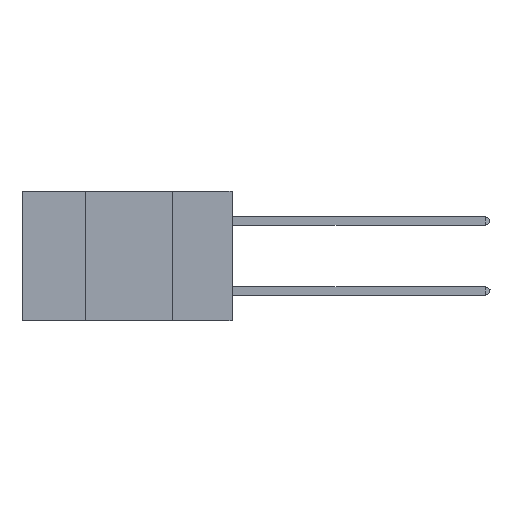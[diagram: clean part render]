
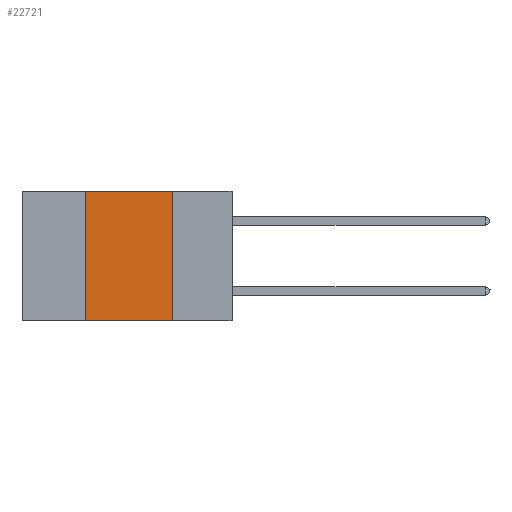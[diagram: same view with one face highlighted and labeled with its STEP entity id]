
A CAD part, left-side view. The second image highlights one B-rep face of the part: STEP entity #22721.
In plain terms, the highlighted planar face has unit normal (-1, 0, 0).
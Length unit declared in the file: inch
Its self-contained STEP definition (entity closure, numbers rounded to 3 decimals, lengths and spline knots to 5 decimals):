
#283 = PLANE ( 'NONE',  #12346 ) ;
#873 = DIRECTION ( 'NONE',  ( 0., 0., -1. ) ) ;
#2026 = VECTOR ( 'NONE', #14570, 39.37008 ) ;
#3414 = VERTEX_POINT ( 'NONE', #14334 ) ;
#3845 = ORIENTED_EDGE ( 'NONE', *, *, #28315, .F. ) ;
#4107 = ORIENTED_EDGE ( 'NONE', *, *, #23686, .F. ) ;
#4733 = CARTESIAN_POINT ( 'NONE',  ( 0., 0.6, 0. ) ) ;
#4884 = EDGE_CURVE ( 'NONE', #3414, #23263, #25517, .T. ) ;
#5746 = DIRECTION ( 'NONE',  ( 0., 0., 1. ) ) ;
#6227 = CARTESIAN_POINT ( 'NONE',  ( 0., 0.17, 0. ) ) ;
#6267 = VECTOR ( 'NONE', #20473, 39.37008 ) ;
#7265 = CARTESIAN_POINT ( 'NONE',  ( 0., 0.17, -0.37 ) ) ;
#7806 = LINE ( 'NONE', #25553, #24580 ) ;
#7925 = ORIENTED_EDGE ( 'NONE', *, *, #22971, .T. ) ;
#9205 = DIRECTION ( 'NONE',  ( 1., 0., 0. ) ) ;
#10500 = LINE ( 'NONE', #23168, #2026 ) ;
#12346 = AXIS2_PLACEMENT_3D ( 'NONE', #23023, #9205, #873 ) ;
#14334 = CARTESIAN_POINT ( 'NONE',  ( 0., 0.17, 0. ) ) ;
#14570 = DIRECTION ( 'NONE',  ( 0., -1., 0. ) ) ;
#18071 = FACE_OUTER_BOUND ( 'NONE', #26517, .T. ) ;
#19917 = DIRECTION ( 'NONE',  ( 0., 0., -1. ) ) ;
#20473 = DIRECTION ( 'NONE',  ( 0., -1., 0. ) ) ;
#22721 = ADVANCED_FACE ( 'NONE', ( #18071 ), #283, .F. ) ;
#22971 = EDGE_CURVE ( 'NONE', #26124, #23263, #10500, .T. ) ;
#23023 = CARTESIAN_POINT ( 'NONE',  ( 0., 0.6, 0. ) ) ;
#23168 = CARTESIAN_POINT ( 'NONE',  ( 0., 0.6, -0.37 ) ) ;
#23263 = VERTEX_POINT ( 'NONE', #7265 ) ;
#23364 = ORIENTED_EDGE ( 'NONE', *, *, #4884, .F. ) ;
#23686 = EDGE_CURVE ( 'NONE', #27716, #3414, #24550, .T. ) ;
#24491 = VECTOR ( 'NONE', #19917, 39.37008 ) ;
#24550 = LINE ( 'NONE', #4733, #6267 ) ;
#24580 = VECTOR ( 'NONE', #5746, 39.37008 ) ;
#25517 = LINE ( 'NONE', #6227, #24491 ) ;
#25553 = CARTESIAN_POINT ( 'NONE',  ( 0., 0.42, 0. ) ) ;
#25761 = CARTESIAN_POINT ( 'NONE',  ( 0., 0.42, -0.37 ) ) ;
#26124 = VERTEX_POINT ( 'NONE', #25761 ) ;
#26517 = EDGE_LOOP ( 'NONE', ( #23364, #4107, #3845, #7925 ) ) ;
#27056 = CARTESIAN_POINT ( 'NONE',  ( 0., 0.42, 0. ) ) ;
#27716 = VERTEX_POINT ( 'NONE', #27056 ) ;
#28315 = EDGE_CURVE ( 'NONE', #26124, #27716, #7806, .T. ) ;
